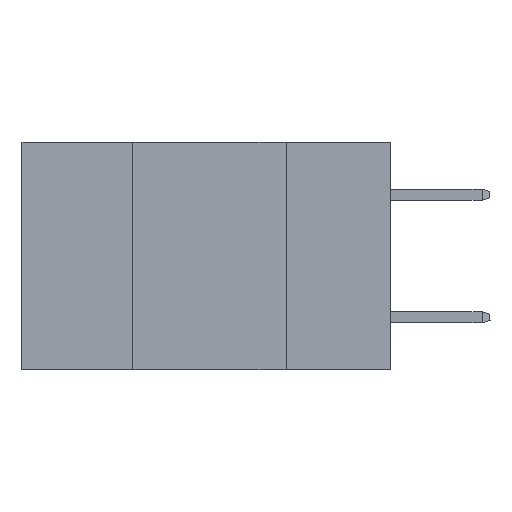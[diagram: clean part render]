
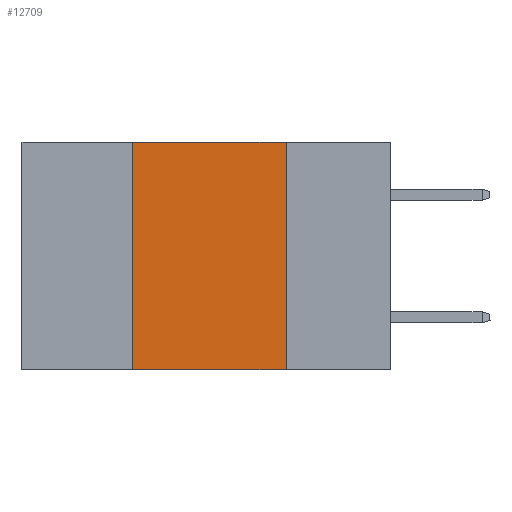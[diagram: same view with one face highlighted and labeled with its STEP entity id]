
A CAD part, left-side view. The second image highlights one B-rep face of the part: STEP entity #12709.
In plain terms, the highlighted planar face has unit normal (-1, 0, 0).
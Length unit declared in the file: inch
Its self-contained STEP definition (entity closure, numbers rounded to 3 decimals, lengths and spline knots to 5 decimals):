
#826 = LINE ( 'NONE', #9499, #1155 ) ;
#1155 = VECTOR ( 'NONE', #25195, 39.37008 ) ;
#2811 = LINE ( 'NONE', #25399, #25580 ) ;
#4280 = ORIENTED_EDGE ( 'NONE', *, *, #11764, .F. ) ;
#5677 = CARTESIAN_POINT ( 'NONE',  ( 0., 0.17, 0. ) ) ;
#6027 = DIRECTION ( 'NONE',  ( 1., 0., 0. ) ) ;
#6324 = AXIS2_PLACEMENT_3D ( 'NONE', #14889, #6027, #21431 ) ;
#6836 = DIRECTION ( 'NONE',  ( 0., 0., -1. ) ) ;
#7023 = EDGE_LOOP ( 'NONE', ( #22926, #14129, #4280, #23876 ) ) ;
#7836 = DIRECTION ( 'NONE',  ( 0., -1., 0. ) ) ;
#8333 = CARTESIAN_POINT ( 'NONE',  ( 0., 0.42, 0. ) ) ;
#8334 = CARTESIAN_POINT ( 'NONE',  ( 0., 0.42, -0.37 ) ) ;
#9499 = CARTESIAN_POINT ( 'NONE',  ( 0., 0.42, 0. ) ) ;
#9749 = DIRECTION ( 'NONE',  ( 0., -1., 0. ) ) ;
#10060 = VERTEX_POINT ( 'NONE', #8334 ) ;
#11361 = CARTESIAN_POINT ( 'NONE',  ( 0., 0.17, 0. ) ) ;
#11764 = EDGE_CURVE ( 'NONE', #10060, #22208, #826, .T. ) ;
#12709 = ADVANCED_FACE ( 'NONE', ( #26268 ), #14986, .F. ) ;
#14129 = ORIENTED_EDGE ( 'NONE', *, *, #18738, .F. ) ;
#14743 = LINE ( 'NONE', #11361, #20585 ) ;
#14889 = CARTESIAN_POINT ( 'NONE',  ( 0., 0.6, 0. ) ) ;
#14986 = PLANE ( 'NONE',  #6324 ) ;
#15202 = VERTEX_POINT ( 'NONE', #5677 ) ;
#15782 = LINE ( 'NONE', #27194, #18521 ) ;
#18494 = CARTESIAN_POINT ( 'NONE',  ( 0., 0.17, -0.37 ) ) ;
#18521 = VECTOR ( 'NONE', #9749, 39.37008 ) ;
#18738 = EDGE_CURVE ( 'NONE', #22208, #15202, #15782, .T. ) ;
#20585 = VECTOR ( 'NONE', #6836, 39.37008 ) ;
#20867 = VERTEX_POINT ( 'NONE', #18494 ) ;
#21431 = DIRECTION ( 'NONE',  ( 0., 0., -1. ) ) ;
#22163 = EDGE_CURVE ( 'NONE', #10060, #20867, #2811, .T. ) ;
#22208 = VERTEX_POINT ( 'NONE', #8333 ) ;
#22926 = ORIENTED_EDGE ( 'NONE', *, *, #28380, .F. ) ;
#23876 = ORIENTED_EDGE ( 'NONE', *, *, #22163, .T. ) ;
#25195 = DIRECTION ( 'NONE',  ( 0., 0., 1. ) ) ;
#25399 = CARTESIAN_POINT ( 'NONE',  ( 0., 0.6, -0.37 ) ) ;
#25580 = VECTOR ( 'NONE', #7836, 39.37008 ) ;
#26268 = FACE_OUTER_BOUND ( 'NONE', #7023, .T. ) ;
#27194 = CARTESIAN_POINT ( 'NONE',  ( 0., 0.6, 0. ) ) ;
#28380 = EDGE_CURVE ( 'NONE', #15202, #20867, #14743, .T. ) ;
